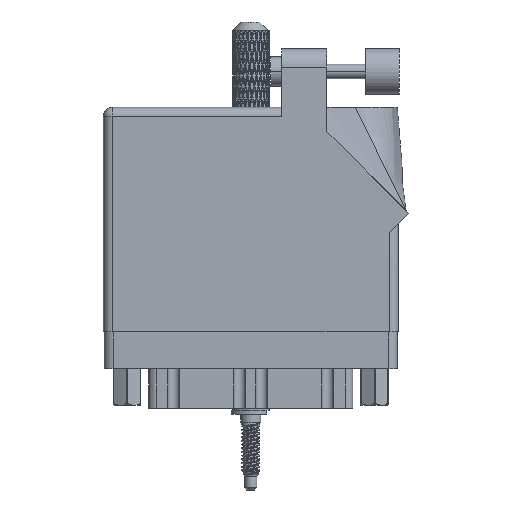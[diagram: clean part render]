
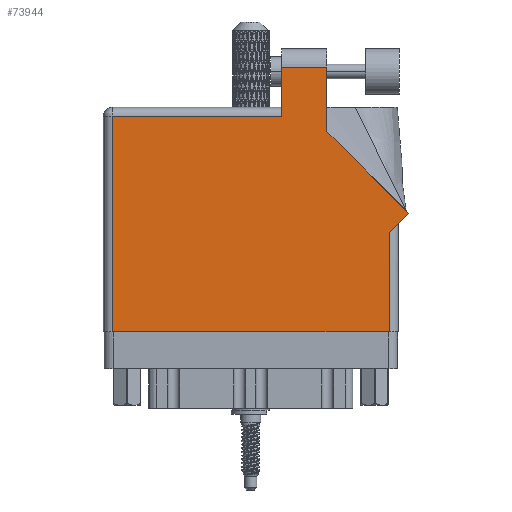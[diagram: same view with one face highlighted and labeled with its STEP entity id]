
A CAD part, front view. The second image highlights one B-rep face of the part: STEP entity #73944.
In plain terms, the highlighted face is planar.
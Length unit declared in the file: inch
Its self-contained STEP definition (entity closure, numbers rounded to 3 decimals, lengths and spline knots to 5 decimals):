
#2163 = ORIENTED_EDGE ( 'NONE', *, *, #59079, .T. ) ;
#2518 = LINE ( 'NONE', #9391, #49947 ) ;
#3163 = EDGE_LOOP ( 'NONE', ( #78737, #70903, #62027, #109088, #41900, #108812, #2163, #19455, #43222 ) ) ;
#4150 = CARTESIAN_POINT ( 'NONE',  ( 2.01, 0.737, 0. ) ) ;
#4502 = DIRECTION ( 'NONE',  ( 0., 1., 0. ) ) ;
#4925 = DIRECTION ( 'NONE',  ( 0., -1., 0. ) ) ;
#7079 = FACE_OUTER_BOUND ( 'NONE', #3163, .T. ) ;
#7859 = EDGE_CURVE ( 'NONE', #69630, #83056, #90973, .T. ) ;
#7928 = VERTEX_POINT ( 'NONE', #32518 ) ;
#8761 = CARTESIAN_POINT ( 'NONE',  ( 0., 0., 0. ) ) ;
#9391 = CARTESIAN_POINT ( 'NONE',  ( 1.948, 0.737, 0. ) ) ;
#11688 = VERTEX_POINT ( 'NONE', #47241 ) ;
#16233 = DIRECTION ( 'NONE',  ( 1., 0., 0. ) ) ;
#19455 = ORIENTED_EDGE ( 'NONE', *, *, #41367, .T. ) ;
#25705 = VECTOR ( 'NONE', #74012, 39.37008 ) ;
#26208 = CARTESIAN_POINT ( 'NONE',  ( 1.948, 0., 0. ) ) ;
#32518 = CARTESIAN_POINT ( 'NONE',  ( 1.948, 0.675, 0. ) ) ;
#33885 = AXIS2_PLACEMENT_3D ( 'NONE', #95281, #48883, #67231 ) ;
#34681 = CARTESIAN_POINT ( 'NONE',  ( 2.08071, 0.80771, 0. ) ) ;
#35331 = EDGE_CURVE ( 'NONE', #111440, #108774, #109146, .T. ) ;
#36071 = CARTESIAN_POINT ( 'NONE',  ( 1.217, 1.805, 0. ) ) ;
#39725 = EDGE_CURVE ( 'NONE', #83056, #61221, #60017, .T. ) ;
#41041 = CARTESIAN_POINT ( 'NONE',  ( 1.524, 1.805, 0. ) ) ;
#41367 = EDGE_CURVE ( 'NONE', #7928, #70377, #102010, .T. ) ;
#41900 = ORIENTED_EDGE ( 'NONE', *, *, #35331, .T. ) ;
#42385 = CARTESIAN_POINT ( 'NONE',  ( 0.062, 0., 0. ) ) ;
#43222 = ORIENTED_EDGE ( 'NONE', *, *, #104452, .T. ) ;
#44976 = CARTESIAN_POINT ( 'NONE',  ( 1.217, 1.53, 0. ) ) ;
#47241 = CARTESIAN_POINT ( 'NONE',  ( 1.217, 1.468, 0. ) ) ;
#48883 = DIRECTION ( 'NONE',  ( 0., 0., -1. ) ) ;
#49947 = VECTOR ( 'NONE', #97017, 39.37008 ) ;
#51349 = VECTOR ( 'NONE', #86350, 39.37008 ) ;
#52831 = EDGE_CURVE ( 'NONE', #11688, #111440, #60410, .T. ) ;
#53522 = CARTESIAN_POINT ( 'NONE',  ( 1.524, 1.36442, 0. ) ) ;
#55339 = CARTESIAN_POINT ( 'NONE',  ( 0.062, 1.468, 0. ) ) ;
#57790 = EDGE_CURVE ( 'NONE', #61221, #11688, #108980, .T. ) ;
#58287 = VECTOR ( 'NONE', #4925, 39.37008 ) ;
#59079 = EDGE_CURVE ( 'NONE', #69312, #7928, #2518, .T. ) ;
#60017 = LINE ( 'NONE', #96648, #51349 ) ;
#60410 = LINE ( 'NONE', #95353, #87296 ) ;
#61221 = VERTEX_POINT ( 'NONE', #36071 ) ;
#62027 = ORIENTED_EDGE ( 'NONE', *, *, #57790, .T. ) ;
#63541 = EDGE_CURVE ( 'NONE', #108774, #69312, #86658, .T. ) ;
#64675 = VECTOR ( 'NONE', #4502, 39.37008 ) ;
#65442 = DIRECTION ( 'NONE',  ( 0., -1., 0. ) ) ;
#66666 = PLANE ( 'NONE',  #33885 ) ;
#67231 = DIRECTION ( 'NONE',  ( -1., 0., 0. ) ) ;
#67785 = CARTESIAN_POINT ( 'NONE',  ( 2.08071, 0.80771, 0. ) ) ;
#69312 = VERTEX_POINT ( 'NONE', #26208 ) ;
#69630 = VERTEX_POINT ( 'NONE', #53522 ) ;
#70377 = VERTEX_POINT ( 'NONE', #34681 ) ;
#70903 = ORIENTED_EDGE ( 'NONE', *, *, #39725, .T. ) ;
#73944 = ADVANCED_FACE ( 'NONE', ( #7079 ), #66666, .F. ) ;
#74012 = DIRECTION ( 'NONE',  ( 0.707, 0.707, 0. ) ) ;
#78737 = ORIENTED_EDGE ( 'NONE', *, *, #7859, .T. ) ;
#79283 = VECTOR ( 'NONE', #16233, 39.37008 ) ;
#82940 = CARTESIAN_POINT ( 'NONE',  ( 1.524, 1.36442, 0. ) ) ;
#83056 = VERTEX_POINT ( 'NONE', #41041 ) ;
#85518 = DIRECTION ( 'NONE',  ( -0.707, 0.707, 0. ) ) ;
#86350 = DIRECTION ( 'NONE',  ( -1., 0., 0. ) ) ;
#86658 = LINE ( 'NONE', #8761, #79283 ) ;
#86761 = DIRECTION ( 'NONE',  ( -1., 0., 0. ) ) ;
#87296 = VECTOR ( 'NONE', #86761, 39.37008 ) ;
#87573 = VECTOR ( 'NONE', #85518, 39.37008 ) ;
#90973 = LINE ( 'NONE', #82940, #64675 ) ;
#95281 = CARTESIAN_POINT ( 'NONE',  ( 0., 1.53, 0. ) ) ;
#95353 = CARTESIAN_POINT ( 'NONE',  ( 0., 1.468, 0. ) ) ;
#96648 = CARTESIAN_POINT ( 'NONE',  ( 1.217, 1.805, 0. ) ) ;
#97017 = DIRECTION ( 'NONE',  ( 0., 1., 0. ) ) ;
#102010 = LINE ( 'NONE', #4150, #25705 ) ;
#104452 = EDGE_CURVE ( 'NONE', #70377, #69630, #111880, .T. ) ;
#108591 = CARTESIAN_POINT ( 'NONE',  ( 0.062, 0., 0. ) ) ;
#108774 = VERTEX_POINT ( 'NONE', #42385 ) ;
#108812 = ORIENTED_EDGE ( 'NONE', *, *, #63541, .T. ) ;
#108980 = LINE ( 'NONE', #44976, #110227 ) ;
#109088 = ORIENTED_EDGE ( 'NONE', *, *, #52831, .T. ) ;
#109146 = LINE ( 'NONE', #108591, #58287 ) ;
#110227 = VECTOR ( 'NONE', #65442, 39.37008 ) ;
#111440 = VERTEX_POINT ( 'NONE', #55339 ) ;
#111880 = LINE ( 'NONE', #67785, #87573 ) ;
